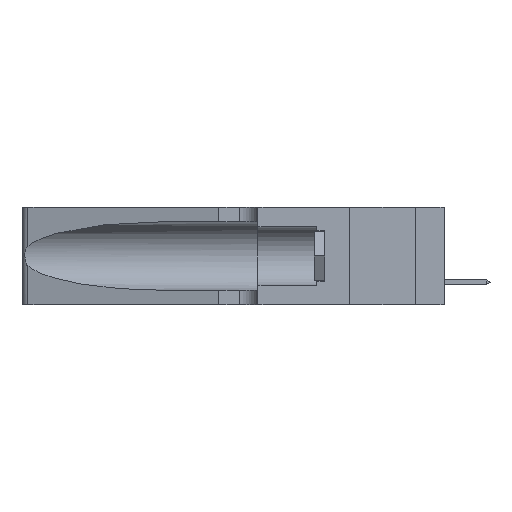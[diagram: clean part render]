
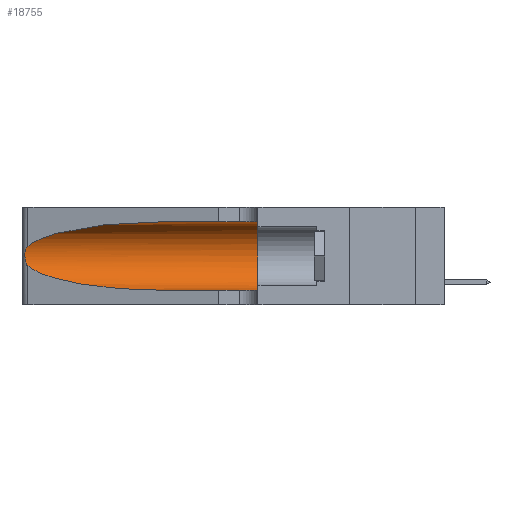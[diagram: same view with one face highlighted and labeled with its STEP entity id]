
A CAD part, left-side view. The second image highlights one B-rep face of the part: STEP entity #18755.
In plain terms, the highlighted cylindrical face has radius 3.308 mm (diameter 6.617 mm), a partial arc.
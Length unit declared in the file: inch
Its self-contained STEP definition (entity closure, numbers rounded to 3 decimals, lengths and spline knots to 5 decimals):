
#1706 =( BOUNDED_CURVE ( )  B_SPLINE_CURVE ( 3, ( #29038, #29178, #4811, #32304 ),
 .UNSPECIFIED., .F., .F. ) 
 B_SPLINE_CURVE_WITH_KNOTS ( ( 4, 4 ),
 ( 3.44316, 4.71239 ),
 .UNSPECIFIED. ) 
 CURVE ( )  GEOMETRIC_REPRESENTATION_ITEM ( )  RATIONAL_B_SPLINE_CURVE ( ( 1., 0.87, 0.87, 1. ) ) 
 REPRESENTATION_ITEM ( '' )  );
#2858 = ORIENTED_EDGE ( 'NONE', *, *, #4572, .T. ) ;
#3961 = CARTESIAN_POINT ( 'NONE',  ( 0.25487, 1.22718, 0.22369 ) ) ;
#4423 = VERTEX_POINT ( 'NONE', #33329 ) ;
#4572 = EDGE_CURVE ( 'NONE', #4423, #23059, #28704, .T. ) ;
#4690 = EDGE_CURVE ( 'NONE', #10706, #28643, #21575, .T. ) ;
#4811 = CARTESIAN_POINT ( 'NONE',  ( 0.18966, 0.96281, 0.05475 ) ) ;
#5215 = CARTESIAN_POINT ( 'NONE',  ( 0.25854, 1.2359, 0.20912 ) ) ;
#5226 = CIRCLE ( 'NONE', #14267, 0.13025 ) ;
#5342 = CARTESIAN_POINT ( 'NONE',  ( 0.26075, 1.23896, 0.178 ) ) ;
#5623 = DIRECTION ( 'NONE',  ( 0., -1., 0. ) ) ;
#6849 = EDGE_CURVE ( 'NONE', #26155, #10706, #17377, .T. ) ;
#7133 = EDGE_CURVE ( 'NONE', #38562, #23059, #5226, .T. ) ;
#7851 = ORIENTED_EDGE ( 'NONE', *, *, #37306, .F. ) ;
#8037 = DIRECTION ( 'NONE',  ( 0., 1., 0. ) ) ;
#8225 = CARTESIAN_POINT ( 'NONE',  ( 0.25787, 1.23484, 0.2124 ) ) ;
#8957 = CARTESIAN_POINT ( 'NONE',  ( 0.1305, 0.35, 0.05475 ) ) ;
#9284 = CARTESIAN_POINT ( 'NONE',  ( 0.1305, 0.72297, 0.31525 ) ) ;
#9686 = CARTESIAN_POINT ( 'NONE',  ( 0.25555, 1.22993, 0.14849 ) ) ;
#9931 = CARTESIAN_POINT ( 'NONE',  ( 0.25487, 1.22718, 0.14631 ) ) ;
#10318 = VECTOR ( 'NONE', #5623, 39.37008 ) ;
#10706 = VERTEX_POINT ( 'NONE', #3961 ) ;
#11084 = ORIENTED_EDGE ( 'NONE', *, *, #16123, .T. ) ;
#12171 = DIRECTION ( 'NONE',  ( 0., -1., 0. ) ) ;
#12807 = DIRECTION ( 'NONE',  ( 0., -1., 0. ) ) ;
#12931 = CYLINDRICAL_SURFACE ( 'NONE', #23881, 0.13025 ) ;
#13168 = CARTESIAN_POINT ( 'NONE',  ( 0.2373, 1.15595, 0.28018 ) ) ;
#14267 = AXIS2_PLACEMENT_3D ( 'NONE', #20851, #8037, #36024 ) ;
#15032 = DIRECTION ( 'NONE',  ( 0., 0., -1. ) ) ;
#15175 = CARTESIAN_POINT ( 'NONE',  ( 0.1305, 1.61858, 0.185 ) ) ;
#15913 = CARTESIAN_POINT ( 'NONE',  ( 0.25487, 1.22718, 0.14631 ) ) ;
#16123 = EDGE_CURVE ( 'NONE', #28643, #4423, #1706, .T. ) ;
#16309 = CARTESIAN_POINT ( 'NONE',  ( 0.25487, 1.22718, 0.22369 ) ) ;
#17377 =( BOUNDED_CURVE ( )  B_SPLINE_CURVE ( 3, ( #9284, #31594, #13168, #16309 ),
 .UNSPECIFIED., .F., .F. ) 
 B_SPLINE_CURVE_WITH_KNOTS ( ( 4, 4 ),
 ( 1.5708, 2.84003 ),
 .UNSPECIFIED. ) 
 CURVE ( )  GEOMETRIC_REPRESENTATION_ITEM ( )  RATIONAL_B_SPLINE_CURVE ( ( 1., 0.87, 0.87, 1. ) ) 
 REPRESENTATION_ITEM ( '' )  );
#18755 = ADVANCED_FACE ( 'NONE', ( #22145 ), #12931, .F. ) ;
#20249 = CARTESIAN_POINT ( 'NONE',  ( 0.25487, 1.22718, 0.22369 ) ) ;
#20851 = CARTESIAN_POINT ( 'NONE',  ( 0.1305, 0.35, 0.185 ) ) ;
#21575 = B_SPLINE_CURVE_WITH_KNOTS ( 'NONE', 3,
 ( #20249, #23367, #32850, #8225, #5215, #33374, #24295, #5342, #30365, #36364, #24015, #31191, #9686, #15913 ),
 .UNSPECIFIED., .F., .F.,
 ( 4, 2, 2, 2, 2, 2, 4 ),
 ( 0., 0.00027, 0.00053, 0.00107, 0.0016, 0.00187, 0.00214 ),
 .UNSPECIFIED. ) ;
#21928 = VECTOR ( 'NONE', #12807, 39.37008 ) ;
#22145 = FACE_OUTER_BOUND ( 'NONE', #38232, .T. ) ;
#22158 = CARTESIAN_POINT ( 'NONE',  ( 0.1305, 1.61858, 0.31525 ) ) ;
#22895 = LINE ( 'NONE', #22158, #21928 ) ;
#23059 = VERTEX_POINT ( 'NONE', #8957 ) ;
#23367 = CARTESIAN_POINT ( 'NONE',  ( 0.25555, 1.22994, 0.2215 ) ) ;
#23881 = AXIS2_PLACEMENT_3D ( 'NONE', #15175, #12171, #15032 ) ;
#23890 = ORIENTED_EDGE ( 'NONE', *, *, #7133, .F. ) ;
#24015 = CARTESIAN_POINT ( 'NONE',  ( 0.25789, 1.23486, 0.15765 ) ) ;
#24169 = CARTESIAN_POINT ( 'NONE',  ( 0.1305, 1.61858, 0.05475 ) ) ;
#24295 = CARTESIAN_POINT ( 'NONE',  ( 0.26075, 1.23896, 0.19203 ) ) ;
#26155 = VERTEX_POINT ( 'NONE', #27485 ) ;
#27485 = CARTESIAN_POINT ( 'NONE',  ( 0.1305, 0.72297, 0.31525 ) ) ;
#28643 = VERTEX_POINT ( 'NONE', #9931 ) ;
#28704 = LINE ( 'NONE', #24169, #10318 ) ;
#29038 = CARTESIAN_POINT ( 'NONE',  ( 0.25487, 1.22718, 0.14631 ) ) ;
#29178 = CARTESIAN_POINT ( 'NONE',  ( 0.2373, 1.15595, 0.08982 ) ) ;
#30365 = CARTESIAN_POINT ( 'NONE',  ( 0.26017, 1.23833, 0.17102 ) ) ;
#31191 = CARTESIAN_POINT ( 'NONE',  ( 0.25639, 1.23186, 0.15144 ) ) ;
#31594 = CARTESIAN_POINT ( 'NONE',  ( 0.18966, 0.96281, 0.31525 ) ) ;
#32304 = CARTESIAN_POINT ( 'NONE',  ( 0.1305, 0.72297, 0.05475 ) ) ;
#32850 = CARTESIAN_POINT ( 'NONE',  ( 0.25639, 1.23184, 0.21858 ) ) ;
#33101 = ORIENTED_EDGE ( 'NONE', *, *, #4690, .T. ) ;
#33329 = CARTESIAN_POINT ( 'NONE',  ( 0.1305, 0.72297, 0.05475 ) ) ;
#33374 = CARTESIAN_POINT ( 'NONE',  ( 0.26018, 1.23835, 0.19895 ) ) ;
#35575 = CARTESIAN_POINT ( 'NONE',  ( 0.1305, 0.35, 0.31525 ) ) ;
#36024 = DIRECTION ( 'NONE',  ( 0., 0., 1. ) ) ;
#36364 = CARTESIAN_POINT ( 'NONE',  ( 0.25856, 1.23593, 0.16098 ) ) ;
#37306 = EDGE_CURVE ( 'NONE', #26155, #38562, #22895, .T. ) ;
#38232 = EDGE_LOOP ( 'NONE', ( #40148, #33101, #11084, #2858, #23890, #7851 ) ) ;
#38562 = VERTEX_POINT ( 'NONE', #35575 ) ;
#40148 = ORIENTED_EDGE ( 'NONE', *, *, #6849, .T. ) ;
